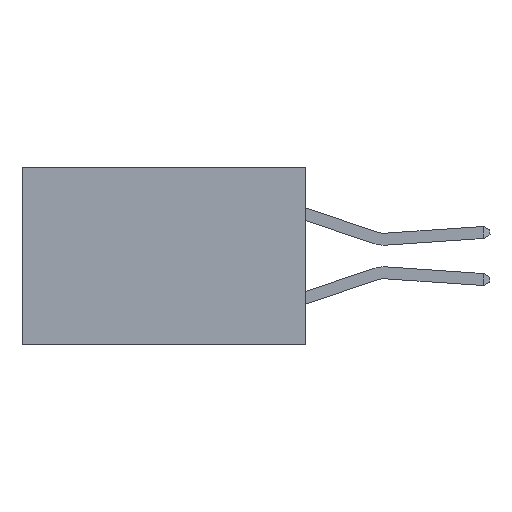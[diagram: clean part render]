
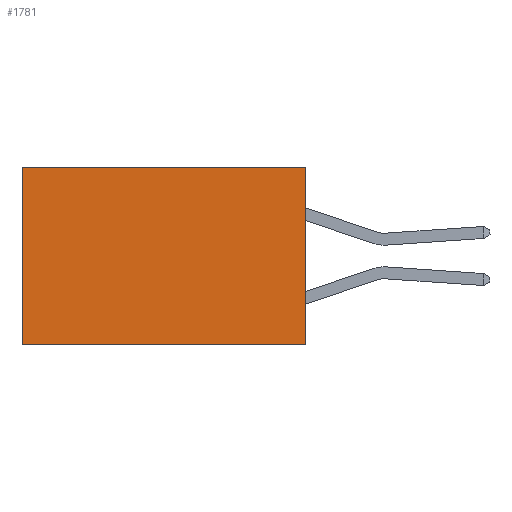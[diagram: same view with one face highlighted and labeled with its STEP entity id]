
A CAD part, left-side view. The second image highlights one B-rep face of the part: STEP entity #1781.
In plain terms, the highlighted planar face has unit normal (-1, 0, 0).
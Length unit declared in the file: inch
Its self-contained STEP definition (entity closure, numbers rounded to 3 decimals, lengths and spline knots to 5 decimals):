
#637 = EDGE_LOOP ( 'NONE', ( #4030, #3950, #3873, #741 ) ) ;
#718 = VECTOR ( 'NONE', #6195, 39.37008 ) ;
#741 = ORIENTED_EDGE ( 'NONE', *, *, #2633, .T. ) ;
#888 = LINE ( 'NONE', #1158, #2912 ) ;
#1009 = FACE_OUTER_BOUND ( 'NONE', #637, .T. ) ;
#1154 = DIRECTION ( 'NONE',  ( 0., 1., 0. ) ) ;
#1158 = CARTESIAN_POINT ( 'NONE',  ( 0.277, 0., 0. ) ) ;
#1179 = VERTEX_POINT ( 'NONE', #5235 ) ;
#1194 = EDGE_CURVE ( 'NONE', #5706, #1179, #2754, .T. ) ;
#1318 = DIRECTION ( 'NONE',  ( 0., 0., -1. ) ) ;
#1781 = ADVANCED_FACE ( 'NONE', ( #1009 ), #4913, .F. ) ;
#2142 = VERTEX_POINT ( 'NONE', #5267 ) ;
#2348 = VECTOR ( 'NONE', #5522, 39.37008 ) ;
#2572 = LINE ( 'NONE', #5373, #2348 ) ;
#2633 = EDGE_CURVE ( 'NONE', #2914, #5706, #888, .T. ) ;
#2754 = LINE ( 'NONE', #7451, #718 ) ;
#2912 = VECTOR ( 'NONE', #1154, 39.37008 ) ;
#2914 = VERTEX_POINT ( 'NONE', #3859 ) ;
#3859 = CARTESIAN_POINT ( 'NONE',  ( 0.277, 0., 0. ) ) ;
#3873 = ORIENTED_EDGE ( 'NONE', *, *, #4118, .F. ) ;
#3950 = ORIENTED_EDGE ( 'NONE', *, *, #6705, .F. ) ;
#4030 = ORIENTED_EDGE ( 'NONE', *, *, #1194, .T. ) ;
#4118 = EDGE_CURVE ( 'NONE', #2914, #2142, #7515, .T. ) ;
#4365 = CARTESIAN_POINT ( 'NONE',  ( 0.277, 0., -0.37 ) ) ;
#4913 = PLANE ( 'NONE',  #5719 ) ;
#5235 = CARTESIAN_POINT ( 'NONE',  ( 0.277, 0.59, -0.37 ) ) ;
#5267 = CARTESIAN_POINT ( 'NONE',  ( 0.277, 0., -0.37 ) ) ;
#5373 = CARTESIAN_POINT ( 'NONE',  ( 0.277, 0., -0.37 ) ) ;
#5376 = DIRECTION ( 'NONE',  ( 1., 0., 0. ) ) ;
#5522 = DIRECTION ( 'NONE',  ( 0., 1., 0. ) ) ;
#5706 = VERTEX_POINT ( 'NONE', #7489 ) ;
#5719 = AXIS2_PLACEMENT_3D ( 'NONE', #4365, #5376, #1318 ) ;
#6051 = VECTOR ( 'NONE', #6467, 39.37008 ) ;
#6195 = DIRECTION ( 'NONE',  ( 0., 0., -1. ) ) ;
#6467 = DIRECTION ( 'NONE',  ( 0., 0., -1. ) ) ;
#6705 = EDGE_CURVE ( 'NONE', #2142, #1179, #2572, .T. ) ;
#7203 = CARTESIAN_POINT ( 'NONE',  ( 0.277, 0., -0.37 ) ) ;
#7451 = CARTESIAN_POINT ( 'NONE',  ( 0.277, 0.59, -0.37 ) ) ;
#7489 = CARTESIAN_POINT ( 'NONE',  ( 0.277, 0.59, 0. ) ) ;
#7515 = LINE ( 'NONE', #7203, #6051 ) ;
